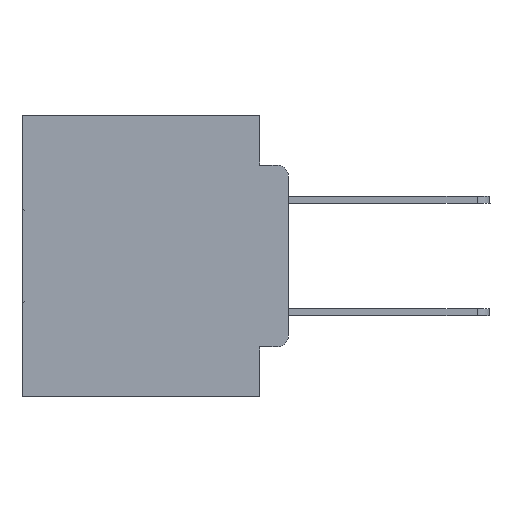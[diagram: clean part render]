
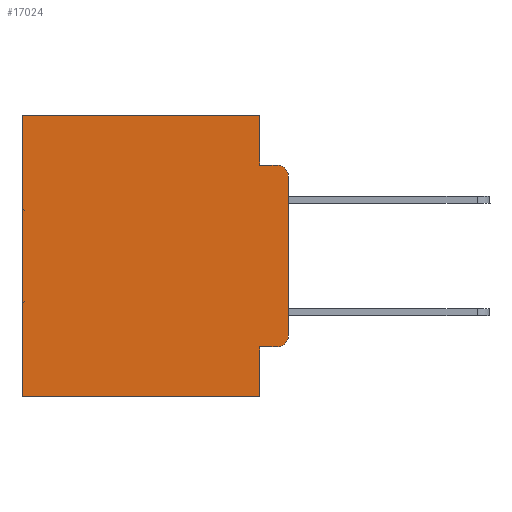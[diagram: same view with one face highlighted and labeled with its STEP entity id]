
A CAD part, left-side view. The second image highlights one B-rep face of the part: STEP entity #17024.
In plain terms, the highlighted planar face has unit normal (-1, 0, 0).
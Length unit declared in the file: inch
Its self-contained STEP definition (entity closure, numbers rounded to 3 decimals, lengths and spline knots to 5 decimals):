
#115 = VERTEX_POINT ( 'NONE', #23696 ) ;
#130 = CARTESIAN_POINT ( 'NONE',  ( 0.298, 0.051, -0.0885 ) ) ;
#426 = CARTESIAN_POINT ( 'NONE',  ( 0.298, 0.051, 0. ) ) ;
#450 = ORIENTED_EDGE ( 'NONE', *, *, #9923, .F. ) ;
#750 = LINE ( 'NONE', #9915, #6692 ) ;
#1468 = EDGE_CURVE ( 'NONE', #6312, #21746, #11519, .T. ) ;
#1634 = VERTEX_POINT ( 'NONE', #17926 ) ;
#2064 = VECTOR ( 'NONE', #17775, 39.37008 ) ;
#2216 = ORIENTED_EDGE ( 'NONE', *, *, #29698, .T. ) ;
#2818 = DIRECTION ( 'NONE',  ( 0., 1., 0. ) ) ;
#2973 = EDGE_LOOP ( 'NONE', ( #13803, #28631, #27771, #450, #2216, #16430, #30000, #8587, #12856, #25612 ) ) ;
#3443 = VERTEX_POINT ( 'NONE', #130 ) ;
#3875 = CARTESIAN_POINT ( 'NONE',  ( 0.298, 0., 0. ) ) ;
#4686 = DIRECTION ( 'NONE',  ( -1., 0., 0. ) ) ;
#4707 = DIRECTION ( 'NONE',  ( 0., 0., -1. ) ) ;
#4902 = CARTESIAN_POINT ( 'NONE',  ( 0.298, 0.02, -0.3915 ) ) ;
#6312 = VERTEX_POINT ( 'NONE', #17336 ) ;
#6690 = LINE ( 'NONE', #15431, #32026 ) ;
#6692 = VECTOR ( 'NONE', #29506, 39.37008 ) ;
#6832 = FACE_OUTER_BOUND ( 'NONE', #2973, .T. ) ;
#7432 = DIRECTION ( 'NONE',  ( 0., 0., -1. ) ) ;
#7501 = DIRECTION ( 'NONE',  ( 0., 0., -1. ) ) ;
#8587 = ORIENTED_EDGE ( 'NONE', *, *, #31823, .F. ) ;
#9915 = CARTESIAN_POINT ( 'NONE',  ( 0.298, 0., 0. ) ) ;
#9923 = EDGE_CURVE ( 'NONE', #27761, #3443, #29137, .T. ) ;
#10085 = DIRECTION ( 'NONE',  ( 0., 1., 0. ) ) ;
#10533 = CIRCLE ( 'NONE', #19344, 0.02 ) ;
#10867 = AXIS2_PLACEMENT_3D ( 'NONE', #4902, #22244, #7432 ) ;
#11341 = AXIS2_PLACEMENT_3D ( 'NONE', #3875, #14014, #31013 ) ;
#11519 = LINE ( 'NONE', #21198, #30238 ) ;
#11602 = EDGE_CURVE ( 'NONE', #3443, #18263, #6690, .T. ) ;
#11941 = CARTESIAN_POINT ( 'NONE',  ( 0.298, 0., 0. ) ) ;
#12856 = ORIENTED_EDGE ( 'NONE', *, *, #30222, .T. ) ;
#12985 = CARTESIAN_POINT ( 'NONE',  ( 0.298, 0., -0.1085 ) ) ;
#13294 = EDGE_CURVE ( 'NONE', #25448, #18263, #10533, .T. ) ;
#13727 = EDGE_CURVE ( 'NONE', #1634, #21746, #30011, .T. ) ;
#13803 = ORIENTED_EDGE ( 'NONE', *, *, #19868, .F. ) ;
#14014 = DIRECTION ( 'NONE',  ( 1., 0., 0. ) ) ;
#14457 = VECTOR ( 'NONE', #7501, 39.37008 ) ;
#14936 = VECTOR ( 'NONE', #29213, 39.37008 ) ;
#15431 = CARTESIAN_POINT ( 'NONE',  ( 0.298, 0.051, -0.0885 ) ) ;
#16430 = ORIENTED_EDGE ( 'NONE', *, *, #1468, .T. ) ;
#17011 = CARTESIAN_POINT ( 'NONE',  ( 0.298, 0.051, -0.4115 ) ) ;
#17024 = ADVANCED_FACE ( 'NONE', ( #6832 ), #23701, .F. ) ;
#17107 = VECTOR ( 'NONE', #2818, 39.37008 ) ;
#17175 = CARTESIAN_POINT ( 'NONE',  ( 0.298, 0.051, 0. ) ) ;
#17336 = CARTESIAN_POINT ( 'NONE',  ( 0.298, 0.473, 0. ) ) ;
#17526 = CARTESIAN_POINT ( 'NONE',  ( 0.298, 0.473, -0.5 ) ) ;
#17619 = LINE ( 'NONE', #11941, #29764 ) ;
#17775 = DIRECTION ( 'NONE',  ( 0., 0., -1. ) ) ;
#17926 = CARTESIAN_POINT ( 'NONE',  ( 0.298, 0.051, -0.5 ) ) ;
#18263 = VERTEX_POINT ( 'NONE', #26480 ) ;
#18557 = CIRCLE ( 'NONE', #10867, 0.02 ) ;
#19344 = AXIS2_PLACEMENT_3D ( 'NONE', #19623, #4686, #22039 ) ;
#19623 = CARTESIAN_POINT ( 'NONE',  ( 0.298, 0.02, -0.1085 ) ) ;
#19868 = EDGE_CURVE ( 'NONE', #25448, #115, #750, .T. ) ;
#20950 = LINE ( 'NONE', #27103, #14457 ) ;
#21198 = CARTESIAN_POINT ( 'NONE',  ( 0.298, 0.473, 0. ) ) ;
#21434 = LINE ( 'NONE', #17011, #14936 ) ;
#21746 = VERTEX_POINT ( 'NONE', #17526 ) ;
#22039 = DIRECTION ( 'NONE',  ( 0., 0., -1. ) ) ;
#22244 = DIRECTION ( 'NONE',  ( -1., 0., 0. ) ) ;
#22299 = VERTEX_POINT ( 'NONE', #28512 ) ;
#23461 = CARTESIAN_POINT ( 'NONE',  ( 0.298, 0.051, -0.4115 ) ) ;
#23696 = CARTESIAN_POINT ( 'NONE',  ( 0.298, 0., -0.3915 ) ) ;
#23701 = PLANE ( 'NONE',  #11341 ) ;
#23720 = EDGE_CURVE ( 'NONE', #22299, #115, #18557, .T. ) ;
#24990 = CARTESIAN_POINT ( 'NONE',  ( 0.298, 0., -0.5 ) ) ;
#25186 = DIRECTION ( 'NONE',  ( 0., -1., 0. ) ) ;
#25448 = VERTEX_POINT ( 'NONE', #12985 ) ;
#25612 = ORIENTED_EDGE ( 'NONE', *, *, #23720, .T. ) ;
#26480 = CARTESIAN_POINT ( 'NONE',  ( 0.298, 0.02, -0.0885 ) ) ;
#27103 = CARTESIAN_POINT ( 'NONE',  ( 0.298, 0.051, 0. ) ) ;
#27761 = VERTEX_POINT ( 'NONE', #17175 ) ;
#27771 = ORIENTED_EDGE ( 'NONE', *, *, #11602, .F. ) ;
#28512 = CARTESIAN_POINT ( 'NONE',  ( 0.298, 0.02, -0.4115 ) ) ;
#28631 = ORIENTED_EDGE ( 'NONE', *, *, #13294, .T. ) ;
#28860 = VERTEX_POINT ( 'NONE', #23461 ) ;
#29137 = LINE ( 'NONE', #426, #2064 ) ;
#29213 = DIRECTION ( 'NONE',  ( 0., -1., 0. ) ) ;
#29506 = DIRECTION ( 'NONE',  ( 0., 0., -1. ) ) ;
#29698 = EDGE_CURVE ( 'NONE', #27761, #6312, #17619, .T. ) ;
#29764 = VECTOR ( 'NONE', #10085, 39.37008 ) ;
#30000 = ORIENTED_EDGE ( 'NONE', *, *, #13727, .F. ) ;
#30011 = LINE ( 'NONE', #24990, #17107 ) ;
#30222 = EDGE_CURVE ( 'NONE', #28860, #22299, #21434, .T. ) ;
#30238 = VECTOR ( 'NONE', #4707, 39.37008 ) ;
#31013 = DIRECTION ( 'NONE',  ( 0., 0., -1. ) ) ;
#31823 = EDGE_CURVE ( 'NONE', #28860, #1634, #20950, .T. ) ;
#32026 = VECTOR ( 'NONE', #25186, 39.37008 ) ;
